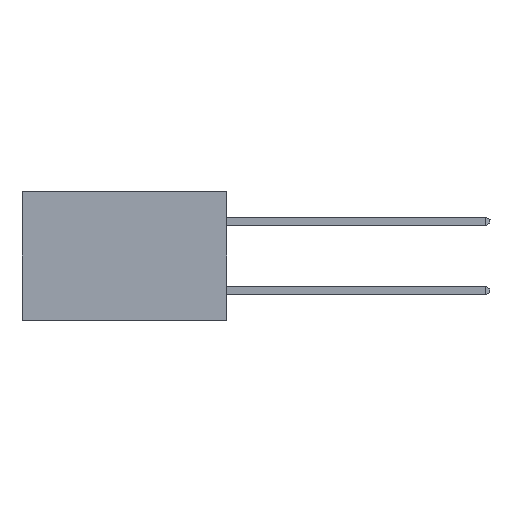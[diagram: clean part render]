
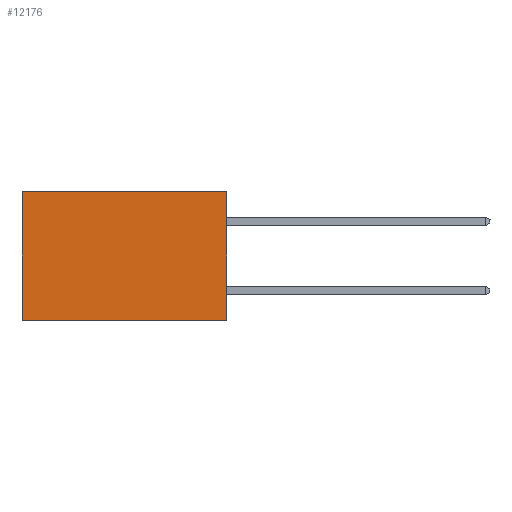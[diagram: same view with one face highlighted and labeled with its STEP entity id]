
A CAD part, left-side view. The second image highlights one B-rep face of the part: STEP entity #12176.
In plain terms, the highlighted planar face has unit normal (-1, 0, 0).
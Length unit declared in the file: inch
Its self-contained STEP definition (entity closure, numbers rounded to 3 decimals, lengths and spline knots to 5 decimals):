
#461 = DIRECTION ( 'NONE',  ( 0., 1., 0. ) ) ;
#1459 = VECTOR ( 'NONE', #15386, 39.37008 ) ;
#1604 = VECTOR ( 'NONE', #461, 39.37008 ) ;
#1827 = FACE_OUTER_BOUND ( 'NONE', #3626, .T. ) ;
#1852 = CARTESIAN_POINT ( 'NONE',  ( 0.277, 0., 0. ) ) ;
#2406 = LINE ( 'NONE', #15494, #1459 ) ;
#3626 = EDGE_LOOP ( 'NONE', ( #9811, #3696, #9546, #6103 ) ) ;
#3658 = LINE ( 'NONE', #4313, #11452 ) ;
#3696 = ORIENTED_EDGE ( 'NONE', *, *, #14556, .F. ) ;
#4313 = CARTESIAN_POINT ( 'NONE',  ( 0.277, 0., -0.37 ) ) ;
#4866 = CARTESIAN_POINT ( 'NONE',  ( 0.277, 0., -0.37 ) ) ;
#5280 = VERTEX_POINT ( 'NONE', #19495 ) ;
#5720 = LINE ( 'NONE', #1852, #1604 ) ;
#5902 = DIRECTION ( 'NONE',  ( 0., 1., 0. ) ) ;
#6103 = ORIENTED_EDGE ( 'NONE', *, *, #11456, .T. ) ;
#6450 = DIRECTION ( 'NONE',  ( 0., 0., -1. ) ) ;
#7682 = EDGE_CURVE ( 'NONE', #19575, #8404, #2406, .T. ) ;
#8113 = CARTESIAN_POINT ( 'NONE',  ( 0.277, 0.59, 0. ) ) ;
#8404 = VERTEX_POINT ( 'NONE', #8448 ) ;
#8448 = CARTESIAN_POINT ( 'NONE',  ( 0.277, 0.59, -0.37 ) ) ;
#9155 = DIRECTION ( 'NONE',  ( 0., 0., -1. ) ) ;
#9546 = ORIENTED_EDGE ( 'NONE', *, *, #10527, .F. ) ;
#9811 = ORIENTED_EDGE ( 'NONE', *, *, #7682, .T. ) ;
#10527 = EDGE_CURVE ( 'NONE', #5280, #15803, #19090, .T. ) ;
#11452 = VECTOR ( 'NONE', #5902, 39.37008 ) ;
#11456 = EDGE_CURVE ( 'NONE', #5280, #19575, #5720, .T. ) ;
#12176 = ADVANCED_FACE ( 'NONE', ( #1827 ), #17251, .F. ) ;
#14556 = EDGE_CURVE ( 'NONE', #15803, #8404, #3658, .T. ) ;
#15327 = CARTESIAN_POINT ( 'NONE',  ( 0.277, 0., -0.37 ) ) ;
#15386 = DIRECTION ( 'NONE',  ( 0., 0., -1. ) ) ;
#15494 = CARTESIAN_POINT ( 'NONE',  ( 0.277, 0.59, -0.37 ) ) ;
#15763 = DIRECTION ( 'NONE',  ( 1., 0., 0. ) ) ;
#15803 = VERTEX_POINT ( 'NONE', #17126 ) ;
#15979 = AXIS2_PLACEMENT_3D ( 'NONE', #4866, #15763, #6450 ) ;
#17126 = CARTESIAN_POINT ( 'NONE',  ( 0.277, 0., -0.37 ) ) ;
#17251 = PLANE ( 'NONE',  #15979 ) ;
#18618 = VECTOR ( 'NONE', #9155, 39.37008 ) ;
#19090 = LINE ( 'NONE', #15327, #18618 ) ;
#19495 = CARTESIAN_POINT ( 'NONE',  ( 0.277, 0., 0. ) ) ;
#19575 = VERTEX_POINT ( 'NONE', #8113 ) ;
